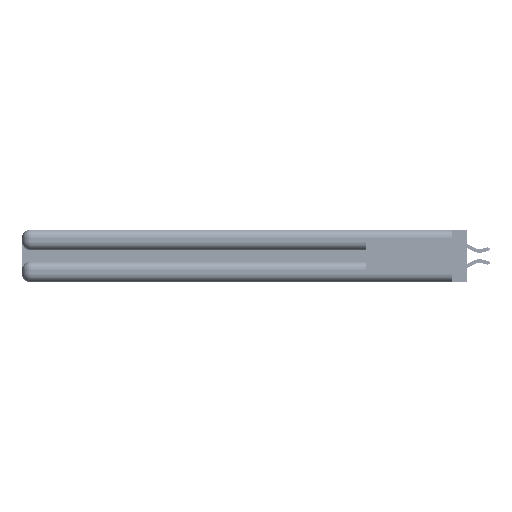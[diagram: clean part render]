
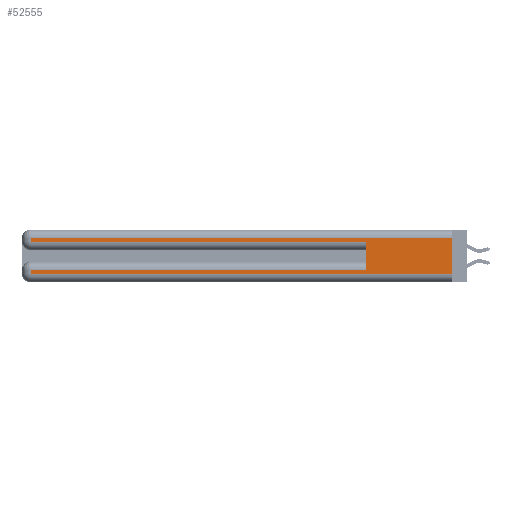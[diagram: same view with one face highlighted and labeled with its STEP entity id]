
A CAD part, left-side view. The second image highlights one B-rep face of the part: STEP entity #52555.
In plain terms, the highlighted planar face has unit normal (-1, 0, 0).
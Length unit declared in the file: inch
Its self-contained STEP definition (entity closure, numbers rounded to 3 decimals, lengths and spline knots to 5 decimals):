
#165 = CARTESIAN_POINT ( 'NONE',  ( 0., 2.94, 0.37 ) ) ;
#1317 = CARTESIAN_POINT ( 'NONE',  ( 0., 2.94, 0.285 ) ) ;
#1459 = ORIENTED_EDGE ( 'NONE', *, *, #17467, .T. ) ;
#6226 = ORIENTED_EDGE ( 'NONE', *, *, #38419, .T. ) ;
#6676 = EDGE_CURVE ( 'NONE', #30783, #48217, #43625, .T. ) ;
#6757 = LINE ( 'NONE', #9215, #38622 ) ;
#9215 = CARTESIAN_POINT ( 'NONE',  ( 0., 0.6, 0.145 ) ) ;
#9316 = LINE ( 'NONE', #50365, #46554 ) ;
#10455 = VERTEX_POINT ( 'NONE', #36910 ) ;
#10676 = VECTOR ( 'NONE', #32958, 39.37008 ) ;
#11006 = CARTESIAN_POINT ( 'NONE',  ( 0., 0., 0.06 ) ) ;
#12643 = ORIENTED_EDGE ( 'NONE', *, *, #45507, .T. ) ;
#12816 = PLANE ( 'NONE',  #48821 ) ;
#13158 = LINE ( 'NONE', #41168, #44357 ) ;
#13770 = DIRECTION ( 'NONE',  ( 0., 0., 1. ) ) ;
#13905 = EDGE_LOOP ( 'NONE', ( #30800, #1459, #33756, #16497, #49492, #12643, #6226, #20954 ) ) ;
#13933 = CARTESIAN_POINT ( 'NONE',  ( 0., 0., 0.37 ) ) ;
#15928 = VERTEX_POINT ( 'NONE', #16527 ) ;
#15950 = VECTOR ( 'NONE', #22281, 39.37008 ) ;
#16129 = VECTOR ( 'NONE', #22127, 39.37008 ) ;
#16497 = ORIENTED_EDGE ( 'NONE', *, *, #41885, .T. ) ;
#16527 = CARTESIAN_POINT ( 'NONE',  ( 0., 2.94, 0.085 ) ) ;
#16694 = CARTESIAN_POINT ( 'NONE',  ( 0., 0., 0.31 ) ) ;
#16802 = VECTOR ( 'NONE', #42118, 39.37008 ) ;
#17354 = CARTESIAN_POINT ( 'NONE',  ( 0., 0., 0.285 ) ) ;
#17467 = EDGE_CURVE ( 'NONE', #28977, #39999, #52000, .T. ) ;
#19578 = DIRECTION ( 'NONE',  ( 0., 0., -1. ) ) ;
#20421 = EDGE_CURVE ( 'NONE', #39999, #36520, #38837, .T. ) ;
#20954 = ORIENTED_EDGE ( 'NONE', *, *, #6676, .T. ) ;
#21886 = VERTEX_POINT ( 'NONE', #37973 ) ;
#22127 = DIRECTION ( 'NONE',  ( 0., 0., -1. ) ) ;
#22281 = DIRECTION ( 'NONE',  ( 0., -1., 0. ) ) ;
#23529 = CARTESIAN_POINT ( 'NONE',  ( 0., 2.94, 0.37 ) ) ;
#25801 = FACE_OUTER_BOUND ( 'NONE', #13905, .T. ) ;
#28679 = VECTOR ( 'NONE', #45852, 39.37008 ) ;
#28977 = VERTEX_POINT ( 'NONE', #16694 ) ;
#30783 = VERTEX_POINT ( 'NONE', #46385 ) ;
#30800 = ORIENTED_EDGE ( 'NONE', *, *, #44202, .F. ) ;
#32750 = DIRECTION ( 'NONE',  ( 0., 1., 0. ) ) ;
#32958 = DIRECTION ( 'NONE',  ( 0., -1., 0. ) ) ;
#33756 = ORIENTED_EDGE ( 'NONE', *, *, #20421, .T. ) ;
#34738 = CARTESIAN_POINT ( 'NONE',  ( 0., 0., 0.06 ) ) ;
#35709 = DIRECTION ( 'NONE',  ( 0., 0., -1. ) ) ;
#35750 = CARTESIAN_POINT ( 'NONE',  ( 0., 2.94, 0.31 ) ) ;
#36520 = VERTEX_POINT ( 'NONE', #1317 ) ;
#36910 = CARTESIAN_POINT ( 'NONE',  ( 0., 0.6, 0.085 ) ) ;
#37194 = CARTESIAN_POINT ( 'NONE',  ( 0., 0., 0.31 ) ) ;
#37973 = CARTESIAN_POINT ( 'NONE',  ( 0., 0.6, 0.285 ) ) ;
#38419 = EDGE_CURVE ( 'NONE', #15928, #30783, #43236, .T. ) ;
#38622 = VECTOR ( 'NONE', #13770, 39.37008 ) ;
#38837 = LINE ( 'NONE', #23529, #28679 ) ;
#39881 = EDGE_CURVE ( 'NONE', #10455, #21886, #6757, .T. ) ;
#39999 = VERTEX_POINT ( 'NONE', #35750 ) ;
#41168 = CARTESIAN_POINT ( 'NONE',  ( 0., 0., 0.37 ) ) ;
#41885 = EDGE_CURVE ( 'NONE', #36520, #21886, #45797, .T. ) ;
#42118 = DIRECTION ( 'NONE',  ( 0., 1., 0. ) ) ;
#43236 = LINE ( 'NONE', #165, #16129 ) ;
#43625 = LINE ( 'NONE', #11006, #10676 ) ;
#43667 = DIRECTION ( 'NONE',  ( 1., 0., 0. ) ) ;
#44202 = EDGE_CURVE ( 'NONE', #28977, #48217, #13158, .T. ) ;
#44357 = VECTOR ( 'NONE', #19578, 39.37008 ) ;
#45507 = EDGE_CURVE ( 'NONE', #10455, #15928, #9316, .T. ) ;
#45797 = LINE ( 'NONE', #17354, #15950 ) ;
#45852 = DIRECTION ( 'NONE',  ( 0., 0., -1. ) ) ;
#46385 = CARTESIAN_POINT ( 'NONE',  ( 0., 2.94, 0.06 ) ) ;
#46554 = VECTOR ( 'NONE', #32750, 39.37008 ) ;
#48217 = VERTEX_POINT ( 'NONE', #34738 ) ;
#48821 = AXIS2_PLACEMENT_3D ( 'NONE', #13933, #43667, #35709 ) ;
#49492 = ORIENTED_EDGE ( 'NONE', *, *, #39881, .F. ) ;
#50365 = CARTESIAN_POINT ( 'NONE',  ( 0., 0., 0.085 ) ) ;
#52000 = LINE ( 'NONE', #37194, #16802 ) ;
#52555 = ADVANCED_FACE ( 'NONE', ( #25801 ), #12816, .F. ) ;
